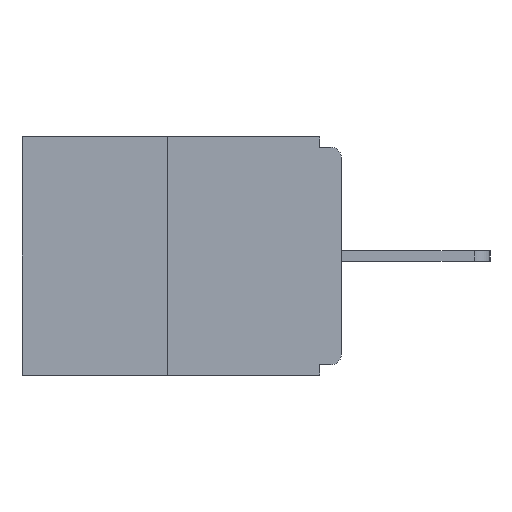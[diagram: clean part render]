
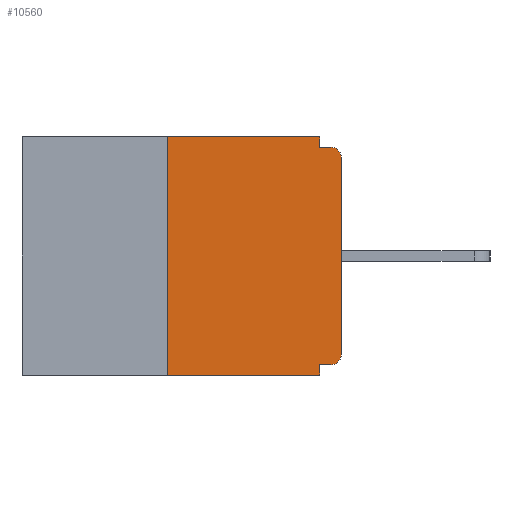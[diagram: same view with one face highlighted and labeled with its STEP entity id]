
A CAD part, left-side view. The second image highlights one B-rep face of the part: STEP entity #10560.
In plain terms, the highlighted planar face has unit normal (-1, 0, 0).
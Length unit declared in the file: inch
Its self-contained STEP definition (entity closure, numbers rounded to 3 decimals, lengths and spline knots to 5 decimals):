
#53 = EDGE_CURVE ( 'NONE', #20202, #444, #3211, .T. ) ;
#146 = PLANE ( 'NONE',  #12470 ) ;
#246 = CARTESIAN_POINT ( 'NONE',  ( 0., 0.031, 0. ) ) ;
#329 = LINE ( 'NONE', #8584, #6157 ) ;
#359 = AXIS2_PLACEMENT_3D ( 'NONE', #17433, #9670, #11030 ) ;
#444 = VERTEX_POINT ( 'NONE', #8762 ) ;
#783 = VECTOR ( 'NONE', #5006, 39.37008 ) ;
#1597 = EDGE_CURVE ( 'NONE', #3296, #19997, #12940, .T. ) ;
#1803 = VECTOR ( 'NONE', #8782, 39.37008 ) ;
#3123 = VERTEX_POINT ( 'NONE', #8276 ) ;
#3211 = LINE ( 'NONE', #8246, #13754 ) ;
#3296 = VERTEX_POINT ( 'NONE', #12244 ) ;
#3991 = ORIENTED_EDGE ( 'NONE', *, *, #1597, .T. ) ;
#4216 = VECTOR ( 'NONE', #5800, 39.37008 ) ;
#4323 = DIRECTION ( 'NONE',  ( 0., 0., 1. ) ) ;
#4565 = CARTESIAN_POINT ( 'NONE',  ( 0., 0.46, 0. ) ) ;
#4848 = CIRCLE ( 'NONE', #6455, 0.015 ) ;
#5006 = DIRECTION ( 'NONE',  ( 0., 0., -1. ) ) ;
#5195 = CARTESIAN_POINT ( 'NONE',  ( 0., 0.015, -0.015 ) ) ;
#5363 = EDGE_CURVE ( 'NONE', #19997, #12526, #4848, .T. ) ;
#5800 = DIRECTION ( 'NONE',  ( 0., 1., 0. ) ) ;
#5922 = EDGE_LOOP ( 'NONE', ( #13442, #19159, #18443, #6888, #18122, #19882, #3991, #6749, #8701, #13438 ) ) ;
#6157 = VECTOR ( 'NONE', #7040, 39.37008 ) ;
#6383 = LINE ( 'NONE', #10644, #4216 ) ;
#6455 = AXIS2_PLACEMENT_3D ( 'NONE', #19609, #10283, #8759 ) ;
#6566 = VECTOR ( 'NONE', #7637, 39.37008 ) ;
#6717 = EDGE_CURVE ( 'NONE', #3123, #3296, #9116, .T. ) ;
#6732 = CARTESIAN_POINT ( 'NONE',  ( 0., 0.46, -0.343 ) ) ;
#6749 = ORIENTED_EDGE ( 'NONE', *, *, #5363, .T. ) ;
#6888 = ORIENTED_EDGE ( 'NONE', *, *, #53, .F. ) ;
#7040 = DIRECTION ( 'NONE',  ( 0., 0., 1. ) ) ;
#7154 = EDGE_CURVE ( 'NONE', #14999, #8033, #19548, .T. ) ;
#7615 = EDGE_CURVE ( 'NONE', #13129, #444, #17591, .T. ) ;
#7637 = DIRECTION ( 'NONE',  ( 0., -1., 0. ) ) ;
#7818 = DIRECTION ( 'NONE',  ( 0., 0., -1. ) ) ;
#7926 = CARTESIAN_POINT ( 'NONE',  ( 0., 0.25, -0.343 ) ) ;
#8033 = VERTEX_POINT ( 'NONE', #246 ) ;
#8246 = CARTESIAN_POINT ( 'NONE',  ( 0., 0.031, -0.343 ) ) ;
#8276 = CARTESIAN_POINT ( 'NONE',  ( 0., 0.015, -0.328 ) ) ;
#8411 = DIRECTION ( 'NONE',  ( 0., -1., 0. ) ) ;
#8545 = CARTESIAN_POINT ( 'NONE',  ( 0., 0.031, -0.015 ) ) ;
#8584 = CARTESIAN_POINT ( 'NONE',  ( 0., 0.25, 0. ) ) ;
#8701 = ORIENTED_EDGE ( 'NONE', *, *, #16672, .F. ) ;
#8759 = DIRECTION ( 'NONE',  ( 0., 0., -1. ) ) ;
#8762 = CARTESIAN_POINT ( 'NONE',  ( 0., 0.031, -0.343 ) ) ;
#8782 = DIRECTION ( 'NONE',  ( 0., -1., 0. ) ) ;
#9116 = CIRCLE ( 'NONE', #359, 0.015 ) ;
#9357 = LINE ( 'NONE', #19016, #783 ) ;
#9620 = LINE ( 'NONE', #16146, #1803 ) ;
#9670 = DIRECTION ( 'NONE',  ( -1., 0., 0. ) ) ;
#10283 = DIRECTION ( 'NONE',  ( -1., 0., 0. ) ) ;
#10560 = ADVANCED_FACE ( 'NONE', ( #17666 ), #146, .F. ) ;
#10644 = CARTESIAN_POINT ( 'NONE',  ( 0., 0., -0.328 ) ) ;
#10918 = DIRECTION ( 'NONE',  ( 1., 0., 0. ) ) ;
#11030 = DIRECTION ( 'NONE',  ( 0., 0., -1. ) ) ;
#11178 = DIRECTION ( 'NONE',  ( 0., 0., -1. ) ) ;
#11705 = CARTESIAN_POINT ( 'NONE',  ( 0., 0.25, 0. ) ) ;
#12244 = CARTESIAN_POINT ( 'NONE',  ( 0., 0., -0.313 ) ) ;
#12470 = AXIS2_PLACEMENT_3D ( 'NONE', #17039, #10918, #7818 ) ;
#12526 = VERTEX_POINT ( 'NONE', #5195 ) ;
#12940 = LINE ( 'NONE', #15187, #17294 ) ;
#12968 = EDGE_CURVE ( 'NONE', #13129, #14999, #329, .T. ) ;
#13129 = VERTEX_POINT ( 'NONE', #7926 ) ;
#13438 = ORIENTED_EDGE ( 'NONE', *, *, #16916, .F. ) ;
#13442 = ORIENTED_EDGE ( 'NONE', *, *, #7154, .F. ) ;
#13754 = VECTOR ( 'NONE', #11178, 39.37008 ) ;
#14999 = VERTEX_POINT ( 'NONE', #11705 ) ;
#15187 = CARTESIAN_POINT ( 'NONE',  ( 0., 0., 0. ) ) ;
#16146 = CARTESIAN_POINT ( 'NONE',  ( 0., 0., -0.015 ) ) ;
#16672 = EDGE_CURVE ( 'NONE', #17456, #12526, #9620, .T. ) ;
#16916 = EDGE_CURVE ( 'NONE', #8033, #17456, #9357, .T. ) ;
#17039 = CARTESIAN_POINT ( 'NONE',  ( 0., 0.46, 0. ) ) ;
#17102 = EDGE_CURVE ( 'NONE', #3123, #20202, #6383, .T. ) ;
#17238 = CARTESIAN_POINT ( 'NONE',  ( 0., 0., -0.03 ) ) ;
#17294 = VECTOR ( 'NONE', #4323, 39.37008 ) ;
#17433 = CARTESIAN_POINT ( 'NONE',  ( 0., 0.015, -0.313 ) ) ;
#17456 = VERTEX_POINT ( 'NONE', #8545 ) ;
#17591 = LINE ( 'NONE', #6732, #18310 ) ;
#17621 = CARTESIAN_POINT ( 'NONE',  ( 0., 0.031, -0.328 ) ) ;
#17666 = FACE_OUTER_BOUND ( 'NONE', #5922, .T. ) ;
#18122 = ORIENTED_EDGE ( 'NONE', *, *, #17102, .F. ) ;
#18310 = VECTOR ( 'NONE', #8411, 39.37008 ) ;
#18443 = ORIENTED_EDGE ( 'NONE', *, *, #7615, .T. ) ;
#19016 = CARTESIAN_POINT ( 'NONE',  ( 0., 0.031, 0. ) ) ;
#19159 = ORIENTED_EDGE ( 'NONE', *, *, #12968, .F. ) ;
#19548 = LINE ( 'NONE', #4565, #6566 ) ;
#19609 = CARTESIAN_POINT ( 'NONE',  ( 0., 0.015, -0.03 ) ) ;
#19882 = ORIENTED_EDGE ( 'NONE', *, *, #6717, .T. ) ;
#19997 = VERTEX_POINT ( 'NONE', #17238 ) ;
#20202 = VERTEX_POINT ( 'NONE', #17621 ) ;
